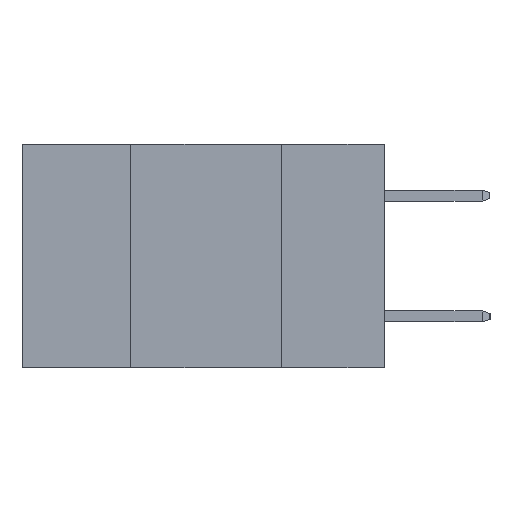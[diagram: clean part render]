
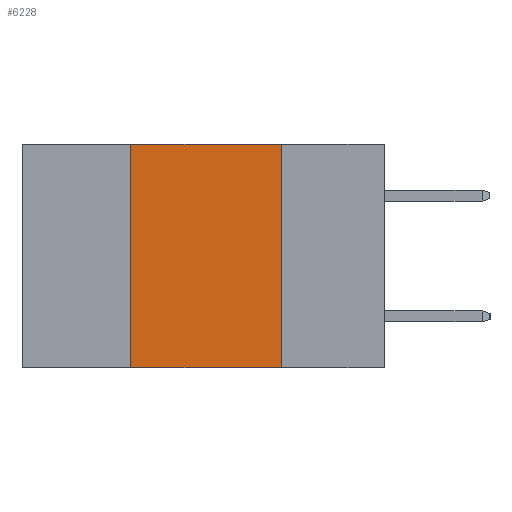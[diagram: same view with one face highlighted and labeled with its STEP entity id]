
A CAD part, left-side view. The second image highlights one B-rep face of the part: STEP entity #6228.
In plain terms, the highlighted planar face has unit normal (-1, 0, 0).
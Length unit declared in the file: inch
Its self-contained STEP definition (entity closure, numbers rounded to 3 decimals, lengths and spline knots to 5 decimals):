
#1164 = VERTEX_POINT ( 'NONE', #11195 ) ;
#1438 = DIRECTION ( 'NONE',  ( 0., 0., 1. ) ) ;
#1563 = EDGE_CURVE ( 'NONE', #4250, #11932, #14995, .T. ) ;
#1576 = CARTESIAN_POINT ( 'NONE',  ( 0., 0.17, -0.37 ) ) ;
#1686 = CARTESIAN_POINT ( 'NONE',  ( 0., 0.17, 0. ) ) ;
#1900 = LINE ( 'NONE', #16101, #5043 ) ;
#3210 = EDGE_CURVE ( 'NONE', #1164, #4250, #9497, .T. ) ;
#3394 = DIRECTION ( 'NONE',  ( 0., 0., -1. ) ) ;
#3449 = DIRECTION ( 'NONE',  ( 1., 0., 0. ) ) ;
#3594 = FACE_OUTER_BOUND ( 'NONE', #11452, .T. ) ;
#3602 = CARTESIAN_POINT ( 'NONE',  ( 0., 0.6, 0. ) ) ;
#3680 = PLANE ( 'NONE',  #6613 ) ;
#3852 = ORIENTED_EDGE ( 'NONE', *, *, #1563, .F. ) ;
#4250 = VERTEX_POINT ( 'NONE', #1686 ) ;
#4518 = CARTESIAN_POINT ( 'NONE',  ( 0., 0.17, -0.37 ) ) ;
#4545 = VECTOR ( 'NONE', #1438, 39.37008 ) ;
#5043 = VECTOR ( 'NONE', #5705, 39.37008 ) ;
#5705 = DIRECTION ( 'NONE',  ( 0., -1., 0. ) ) ;
#5999 = VECTOR ( 'NONE', #12031, 39.37008 ) ;
#6228 = ADVANCED_FACE ( 'NONE', ( #3594 ), #3680, .F. ) ;
#6474 = VERTEX_POINT ( 'NONE', #9616 ) ;
#6613 = AXIS2_PLACEMENT_3D ( 'NONE', #3602, #3449, #3394 ) ;
#7887 = DIRECTION ( 'NONE',  ( 0., 0., -1. ) ) ;
#8618 = EDGE_CURVE ( 'NONE', #6474, #1164, #10780, .T. ) ;
#9212 = ORIENTED_EDGE ( 'NONE', *, *, #8618, .F. ) ;
#9395 = CARTESIAN_POINT ( 'NONE',  ( 0., 0.42, -0.37 ) ) ;
#9497 = LINE ( 'NONE', #12261, #5999 ) ;
#9616 = CARTESIAN_POINT ( 'NONE',  ( 0., 0.42, -0.37 ) ) ;
#10780 = LINE ( 'NONE', #9395, #4545 ) ;
#10880 = ORIENTED_EDGE ( 'NONE', *, *, #12715, .T. ) ;
#11195 = CARTESIAN_POINT ( 'NONE',  ( 0., 0.42, 0. ) ) ;
#11452 = EDGE_LOOP ( 'NONE', ( #3852, #15682, #9212, #10880 ) ) ;
#11932 = VERTEX_POINT ( 'NONE', #1576 ) ;
#12031 = DIRECTION ( 'NONE',  ( 0., -1., 0. ) ) ;
#12261 = CARTESIAN_POINT ( 'NONE',  ( 0., 0.6, 0. ) ) ;
#12715 = EDGE_CURVE ( 'NONE', #6474, #11932, #1900, .T. ) ;
#14075 = VECTOR ( 'NONE', #7887, 39.37008 ) ;
#14995 = LINE ( 'NONE', #4518, #14075 ) ;
#15682 = ORIENTED_EDGE ( 'NONE', *, *, #3210, .F. ) ;
#16101 = CARTESIAN_POINT ( 'NONE',  ( 0., 0.6, -0.37 ) ) ;
